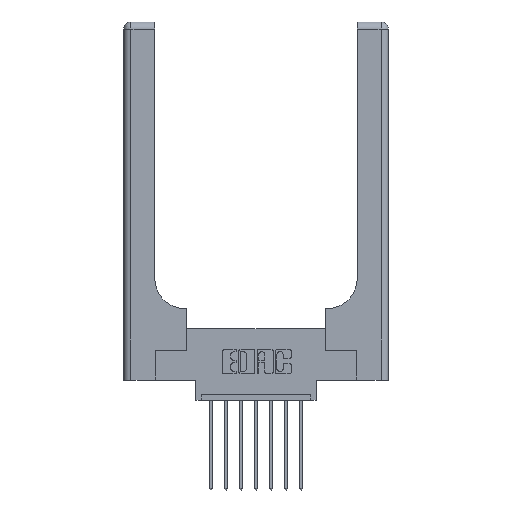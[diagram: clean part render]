
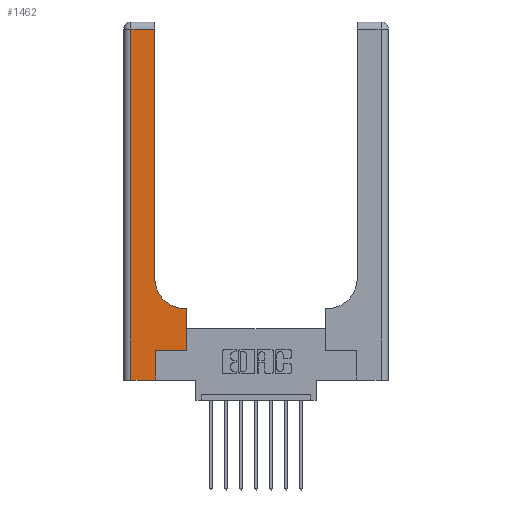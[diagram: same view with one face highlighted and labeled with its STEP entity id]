
A CAD part, top view. The second image highlights one B-rep face of the part: STEP entity #1462.
In plain terms, the highlighted planar face has unit normal (0, 0, 1).
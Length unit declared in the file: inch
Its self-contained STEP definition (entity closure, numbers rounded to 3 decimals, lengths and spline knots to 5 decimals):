
#329 = EDGE_CURVE ( 'NONE', #12059, #3031, #12827, .T. ) ;
#377 = VERTEX_POINT ( 'NONE', #2457 ) ;
#588 = EDGE_CURVE ( 'NONE', #11981, #7529, #9793, .T. ) ;
#614 = LINE ( 'NONE', #1668, #11065 ) ;
#746 = EDGE_CURVE ( 'NONE', #4319, #12059, #6318, .T. ) ;
#1210 = LINE ( 'NONE', #13979, #7183 ) ;
#1275 = FACE_OUTER_BOUND ( 'NONE', #2381, .T. ) ;
#1462 = ADVANCED_FACE ( 'NONE', ( #1275 ), #14417, .F. ) ;
#1668 = CARTESIAN_POINT ( 'NONE',  ( 0.265, 0., 0.37 ) ) ;
#1826 = DIRECTION ( 'NONE',  ( 0., 1., 0. ) ) ;
#1908 = ORIENTED_EDGE ( 'NONE', *, *, #3588, .T. ) ;
#2142 = CARTESIAN_POINT ( 'NONE',  ( 0.06, 2.94, 0.37 ) ) ;
#2232 = ORIENTED_EDGE ( 'NONE', *, *, #8751, .T. ) ;
#2289 = DIRECTION ( 'NONE',  ( 1., 0., 0. ) ) ;
#2381 = EDGE_LOOP ( 'NONE', ( #4740, #1908, #13299, #7080, #8724, #3289, #4408, #2232, #13799 ) ) ;
#2457 = CARTESIAN_POINT ( 'NONE',  ( 0.265, 0.25, 0.37 ) ) ;
#2503 = VECTOR ( 'NONE', #2894, 39.37008 ) ;
#2529 = DIRECTION ( 'NONE',  ( 0., 1., 0. ) ) ;
#2605 = CARTESIAN_POINT ( 'NONE',  ( 0.26, 3., 0.37 ) ) ;
#2894 = DIRECTION ( 'NONE',  ( 1., 0., 0. ) ) ;
#3031 = VERTEX_POINT ( 'NONE', #11565 ) ;
#3289 = ORIENTED_EDGE ( 'NONE', *, *, #12738, .T. ) ;
#3542 = DIRECTION ( 'NONE',  ( 0., 0., -1. ) ) ;
#3588 = EDGE_CURVE ( 'NONE', #3031, #10108, #7556, .T. ) ;
#4195 = DIRECTION ( 'NONE',  ( 0., 0., -1. ) ) ;
#4309 = CARTESIAN_POINT ( 'NONE',  ( 0.265, 0.25, 0.37 ) ) ;
#4319 = VERTEX_POINT ( 'NONE', #13294 ) ;
#4408 = ORIENTED_EDGE ( 'NONE', *, *, #12985, .T. ) ;
#4426 = CARTESIAN_POINT ( 'NONE',  ( 0.265, 0., 0.37 ) ) ;
#4628 = CARTESIAN_POINT ( 'NONE',  ( 0.06, 0., 0.37 ) ) ;
#4740 = ORIENTED_EDGE ( 'NONE', *, *, #329, .T. ) ;
#4761 = VECTOR ( 'NONE', #1826, 39.37008 ) ;
#4944 = AXIS2_PLACEMENT_3D ( 'NONE', #7442, #4195, #13303 ) ;
#6138 = VECTOR ( 'NONE', #6791, 39.37008 ) ;
#6318 = CIRCLE ( 'NONE', #14494, 0.25 ) ;
#6791 = DIRECTION ( 'NONE',  ( -1., 0., 0. ) ) ;
#7074 = VERTEX_POINT ( 'NONE', #12984 ) ;
#7080 = ORIENTED_EDGE ( 'NONE', *, *, #588, .T. ) ;
#7183 = VECTOR ( 'NONE', #8108, 39.37008 ) ;
#7376 = VECTOR ( 'NONE', #12146, 39.37008 ) ;
#7442 = CARTESIAN_POINT ( 'NONE',  ( 0., 3., 0.37 ) ) ;
#7529 = VERTEX_POINT ( 'NONE', #4426 ) ;
#7556 = LINE ( 'NONE', #12080, #7376 ) ;
#8108 = DIRECTION ( 'NONE',  ( 0., -1., 0. ) ) ;
#8462 = CARTESIAN_POINT ( 'NONE',  ( 0.528, 0.6, 0.37 ) ) ;
#8724 = ORIENTED_EDGE ( 'NONE', *, *, #14614, .T. ) ;
#8751 = EDGE_CURVE ( 'NONE', #9565, #4319, #12740, .T. ) ;
#9043 = LINE ( 'NONE', #4309, #10763 ) ;
#9565 = VERTEX_POINT ( 'NONE', #8462 ) ;
#9680 = VECTOR ( 'NONE', #2529, 39.37008 ) ;
#9793 = LINE ( 'NONE', #14518, #2503 ) ;
#10108 = VERTEX_POINT ( 'NONE', #2142 ) ;
#10387 = CARTESIAN_POINT ( 'NONE',  ( 0.51, 0.85, 0.37 ) ) ;
#10496 = CARTESIAN_POINT ( 'NONE',  ( 0.26, 0.85, 0.37 ) ) ;
#10688 = LINE ( 'NONE', #10993, #4761 ) ;
#10763 = VECTOR ( 'NONE', #12359, 39.37008 ) ;
#10993 = CARTESIAN_POINT ( 'NONE',  ( 0.528, 0.25, 0.37 ) ) ;
#11065 = VECTOR ( 'NONE', #14345, 39.37008 ) ;
#11542 = CARTESIAN_POINT ( 'NONE',  ( 0.26, 0.6, 0.37 ) ) ;
#11565 = CARTESIAN_POINT ( 'NONE',  ( 0.26, 2.94, 0.37 ) ) ;
#11981 = VERTEX_POINT ( 'NONE', #4628 ) ;
#12059 = VERTEX_POINT ( 'NONE', #10496 ) ;
#12080 = CARTESIAN_POINT ( 'NONE',  ( 0., 2.94, 0.37 ) ) ;
#12146 = DIRECTION ( 'NONE',  ( -1., 0., 0. ) ) ;
#12359 = DIRECTION ( 'NONE',  ( 1., 0., 0. ) ) ;
#12738 = EDGE_CURVE ( 'NONE', #377, #7074, #9043, .T. ) ;
#12740 = LINE ( 'NONE', #11542, #6138 ) ;
#12827 = LINE ( 'NONE', #2605, #9680 ) ;
#12984 = CARTESIAN_POINT ( 'NONE',  ( 0.528, 0.25, 0.37 ) ) ;
#12985 = EDGE_CURVE ( 'NONE', #7074, #9565, #10688, .T. ) ;
#13260 = EDGE_CURVE ( 'NONE', #10108, #11981, #1210, .T. ) ;
#13294 = CARTESIAN_POINT ( 'NONE',  ( 0.51, 0.6, 0.37 ) ) ;
#13299 = ORIENTED_EDGE ( 'NONE', *, *, #13260, .T. ) ;
#13303 = DIRECTION ( 'NONE',  ( -1., 0., 0. ) ) ;
#13799 = ORIENTED_EDGE ( 'NONE', *, *, #746, .T. ) ;
#13979 = CARTESIAN_POINT ( 'NONE',  ( 0.06, 3., 0.37 ) ) ;
#14345 = DIRECTION ( 'NONE',  ( 0., 1., 0. ) ) ;
#14417 = PLANE ( 'NONE',  #4944 ) ;
#14494 = AXIS2_PLACEMENT_3D ( 'NONE', #10387, #3542, #2289 ) ;
#14518 = CARTESIAN_POINT ( 'NONE',  ( 0., 0., 0.37 ) ) ;
#14614 = EDGE_CURVE ( 'NONE', #7529, #377, #614, .T. ) ;
